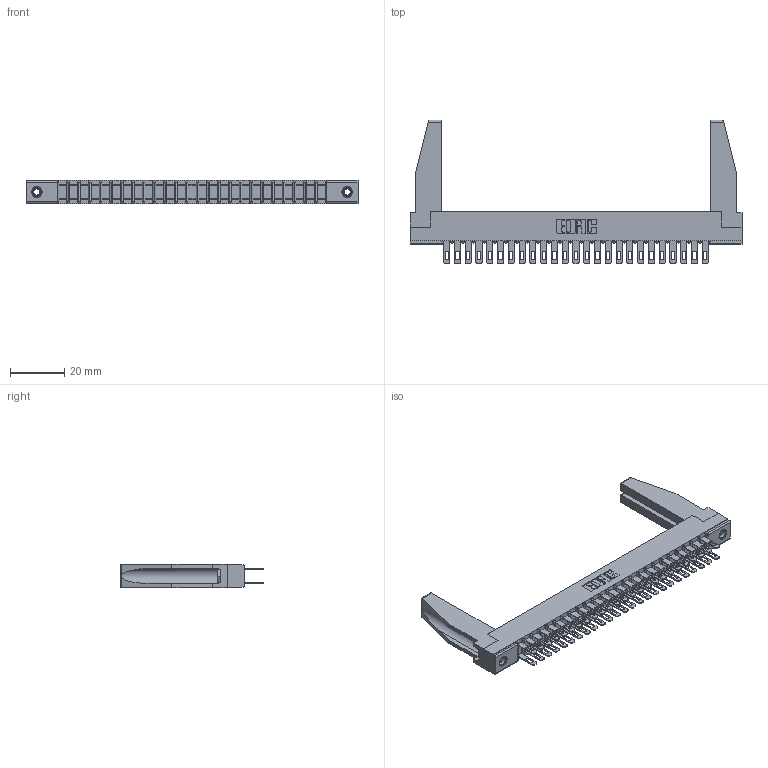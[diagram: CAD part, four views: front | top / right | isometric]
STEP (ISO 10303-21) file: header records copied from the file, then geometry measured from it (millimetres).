
FILE_DESCRIPTION (( 'STEP AP203' ), '1' );
FILE_NAME ('307-050-500-278.STEP', '2019-09-06T10:39:11', ( '' ), ( '' ), 'SwSTEP 2.0', 'SolidWorks 2016', '' );
FILE_SCHEMA (( 'CONFIG_CONTROL_DESIGN' ));
Length unit declared in the file: inch
Products named in the file (5): 307-050-500-278; 345-250-001_345-250-001-102; 307-220-078; 307-290-001_500; 307 Part_.156 Dia Mounting Holes
Assembly tree (55 placements, depth 2):
  307-050-500-278
    307 Part_.156 Dia Mounting Holes
    307-290-001_500  x50
    307-220-078  x2
    345-250-001_345-250-001-102  x2
Bounding box: 122.07 x 52.88 x 8.71 mm (x, y, z)
Volume: 12121.1 mm3; surface area: 19130.9 mm2
Topology: 55 solids, 55 shells, 2574 faces, 7153 edges, 4622 vertices
Faces by surface type: plane 1654, cylinder 852, sphere 52, cone 12, torus 4
Entity records: 26741 total; most frequent: CARTESIAN_POINT 4387, ORIENTED_EDGE 4304, DIRECTION 4260, EDGE_CURVE 2152, VECTOR 1646, LINE 1646, VERTEX_POINT 1392, AXIS2_PLACEMENT_3D 1307
